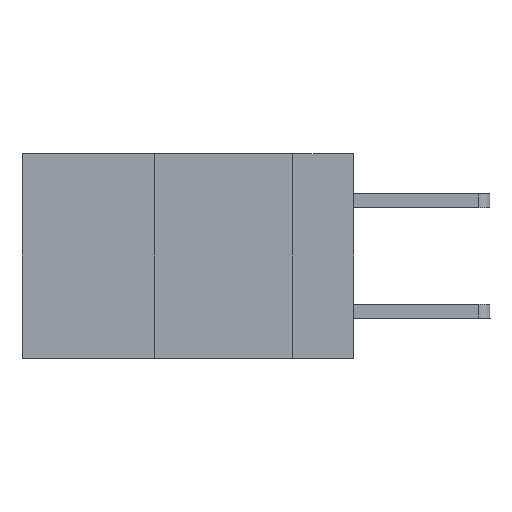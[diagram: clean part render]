
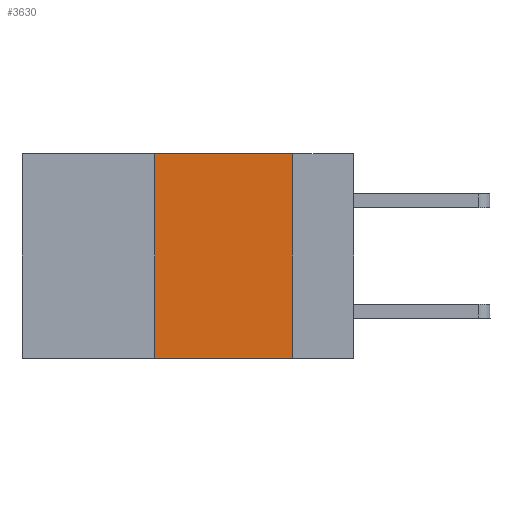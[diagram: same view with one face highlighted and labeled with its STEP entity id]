
A CAD part, left-side view. The second image highlights one B-rep face of the part: STEP entity #3630.
In plain terms, the highlighted planar face has unit normal (-1, 0, 0).
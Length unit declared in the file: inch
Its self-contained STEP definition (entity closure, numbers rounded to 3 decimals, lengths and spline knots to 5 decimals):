
#86 = LINE ( 'NONE', #2837, #3830 ) ;
#119 = CARTESIAN_POINT ( 'NONE',  ( 0., 0.6, -0.37 ) ) ;
#217 = ORIENTED_EDGE ( 'NONE', *, *, #6832, .F. ) ;
#245 = CARTESIAN_POINT ( 'NONE',  ( 0., 0.11, 0. ) ) ;
#458 = LINE ( 'NONE', #8011, #7851 ) ;
#687 = VECTOR ( 'NONE', #7626, 39.37008 ) ;
#818 = DIRECTION ( 'NONE',  ( 0., 0., -1. ) ) ;
#908 = CARTESIAN_POINT ( 'NONE',  ( 0., 0.11, 0. ) ) ;
#1034 = EDGE_CURVE ( 'NONE', #8146, #4424, #86, .T. ) ;
#1368 = VERTEX_POINT ( 'NONE', #3017 ) ;
#2465 = VECTOR ( 'NONE', #818, 39.37008 ) ;
#2803 = DIRECTION ( 'NONE',  ( 0., 0., 1. ) ) ;
#2837 = CARTESIAN_POINT ( 'NONE',  ( 0., 0.36, 0. ) ) ;
#2993 = EDGE_CURVE ( 'NONE', #8146, #1368, #4671, .T. ) ;
#3017 = CARTESIAN_POINT ( 'NONE',  ( 0., 0.11, -0.37 ) ) ;
#3630 = ADVANCED_FACE ( 'NONE', ( #7650 ), #6112, .F. ) ;
#3830 = VECTOR ( 'NONE', #2803, 39.37008 ) ;
#3984 = ORIENTED_EDGE ( 'NONE', *, *, #2993, .T. ) ;
#4098 = DIRECTION ( 'NONE',  ( 0., 0., -1. ) ) ;
#4424 = VERTEX_POINT ( 'NONE', #4436 ) ;
#4436 = CARTESIAN_POINT ( 'NONE',  ( 0., 0.36, 0. ) ) ;
#4525 = DIRECTION ( 'NONE',  ( 0., -1., 0. ) ) ;
#4671 = LINE ( 'NONE', #119, #687 ) ;
#4849 = LINE ( 'NONE', #908, #2465 ) ;
#5390 = ORIENTED_EDGE ( 'NONE', *, *, #8598, .F. ) ;
#5793 = CARTESIAN_POINT ( 'NONE',  ( 0., 0.36, -0.37 ) ) ;
#6112 = PLANE ( 'NONE',  #7257 ) ;
#6253 = EDGE_LOOP ( 'NONE', ( #5390, #217, #7016, #3984 ) ) ;
#6832 = EDGE_CURVE ( 'NONE', #4424, #7464, #458, .T. ) ;
#6876 = DIRECTION ( 'NONE',  ( 1., 0., 0. ) ) ;
#7016 = ORIENTED_EDGE ( 'NONE', *, *, #1034, .F. ) ;
#7257 = AXIS2_PLACEMENT_3D ( 'NONE', #8929, #6876, #4098 ) ;
#7464 = VERTEX_POINT ( 'NONE', #245 ) ;
#7626 = DIRECTION ( 'NONE',  ( 0., -1., 0. ) ) ;
#7650 = FACE_OUTER_BOUND ( 'NONE', #6253, .T. ) ;
#7851 = VECTOR ( 'NONE', #4525, 39.37008 ) ;
#8011 = CARTESIAN_POINT ( 'NONE',  ( 0., 0.6, 0. ) ) ;
#8146 = VERTEX_POINT ( 'NONE', #5793 ) ;
#8598 = EDGE_CURVE ( 'NONE', #7464, #1368, #4849, .T. ) ;
#8929 = CARTESIAN_POINT ( 'NONE',  ( 0., 0.6, 0. ) ) ;
